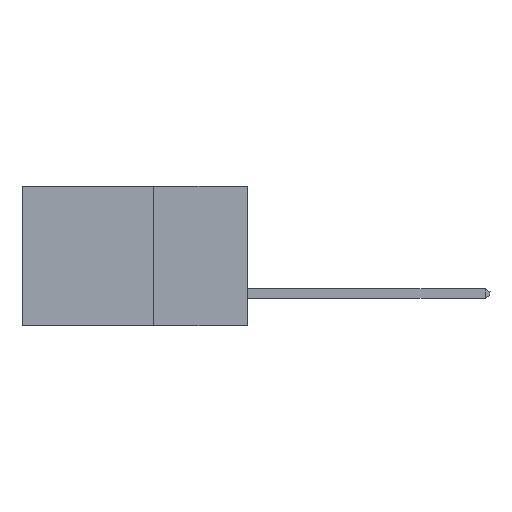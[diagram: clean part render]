
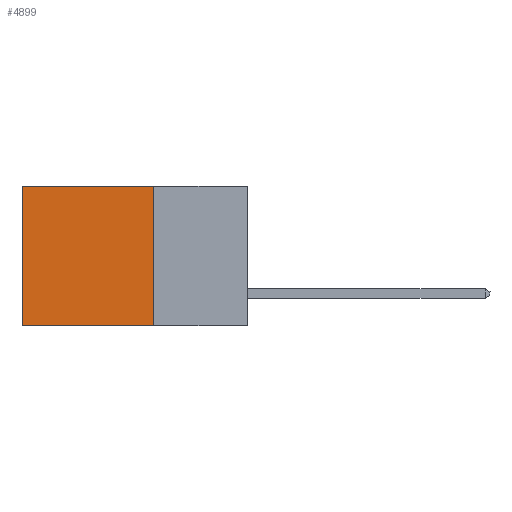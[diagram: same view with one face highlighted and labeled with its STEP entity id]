
A CAD part, left-side view. The second image highlights one B-rep face of the part: STEP entity #4899.
In plain terms, the highlighted planar face has unit normal (-1, 0, 0).
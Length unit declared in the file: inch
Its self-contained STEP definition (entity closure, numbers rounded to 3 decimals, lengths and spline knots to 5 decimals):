
#404 = AXIS2_PLACEMENT_3D ( 'NONE', #7293, #8914, #833 ) ;
#833 = DIRECTION ( 'NONE',  ( 0., 0., -1. ) ) ;
#1270 = CARTESIAN_POINT ( 'NONE',  ( 0.2615, 0.25, 0. ) ) ;
#1564 = FACE_OUTER_BOUND ( 'NONE', #5843, .T. ) ;
#1759 = ORIENTED_EDGE ( 'NONE', *, *, #8696, .T. ) ;
#1832 = VECTOR ( 'NONE', #6645, 39.37008 ) ;
#1913 = ORIENTED_EDGE ( 'NONE', *, *, #4506, .F. ) ;
#1999 = CARTESIAN_POINT ( 'NONE',  ( 0.2615, 0.25, -0.37 ) ) ;
#2515 = EDGE_CURVE ( 'NONE', #5753, #7644, #4645, .T. ) ;
#3374 = EDGE_CURVE ( 'NONE', #5796, #5812, #6791, .T. ) ;
#4292 = VECTOR ( 'NONE', #8492, 39.37008 ) ;
#4506 = EDGE_CURVE ( 'NONE', #5796, #5753, #8198, .T. ) ;
#4645 = LINE ( 'NONE', #7839, #5826 ) ;
#4899 = ADVANCED_FACE ( 'NONE', ( #1564 ), #6525, .F. ) ;
#5390 = DIRECTION ( 'NONE',  ( 0., 0., -1. ) ) ;
#5727 = VECTOR ( 'NONE', #5390, 39.37008 ) ;
#5753 = VERTEX_POINT ( 'NONE', #7578 ) ;
#5796 = VERTEX_POINT ( 'NONE', #1270 ) ;
#5812 = VERTEX_POINT ( 'NONE', #8200 ) ;
#5826 = VECTOR ( 'NONE', #7057, 39.37008 ) ;
#5843 = EDGE_LOOP ( 'NONE', ( #1759, #5981, #1913, #7582 ) ) ;
#5981 = ORIENTED_EDGE ( 'NONE', *, *, #2515, .F. ) ;
#6525 = PLANE ( 'NONE',  #404 ) ;
#6645 = DIRECTION ( 'NONE',  ( 0., 0., -1. ) ) ;
#6746 = CARTESIAN_POINT ( 'NONE',  ( 0.2615, 0.6, -0.37 ) ) ;
#6791 = LINE ( 'NONE', #9162, #4292 ) ;
#6966 = LINE ( 'NONE', #10131, #5727 ) ;
#7057 = DIRECTION ( 'NONE',  ( 0., 1., 0. ) ) ;
#7293 = CARTESIAN_POINT ( 'NONE',  ( 0.2615, 0.25, -0.37 ) ) ;
#7578 = CARTESIAN_POINT ( 'NONE',  ( 0.2615, 0.25, -0.37 ) ) ;
#7582 = ORIENTED_EDGE ( 'NONE', *, *, #3374, .T. ) ;
#7644 = VERTEX_POINT ( 'NONE', #6746 ) ;
#7839 = CARTESIAN_POINT ( 'NONE',  ( 0.2615, 0.25, -0.37 ) ) ;
#8198 = LINE ( 'NONE', #1999, #1832 ) ;
#8200 = CARTESIAN_POINT ( 'NONE',  ( 0.2615, 0.6, 0. ) ) ;
#8492 = DIRECTION ( 'NONE',  ( 0., 1., 0. ) ) ;
#8696 = EDGE_CURVE ( 'NONE', #5812, #7644, #6966, .T. ) ;
#8914 = DIRECTION ( 'NONE',  ( 1., 0., 0. ) ) ;
#9162 = CARTESIAN_POINT ( 'NONE',  ( 0.2615, 0.25, 0. ) ) ;
#10131 = CARTESIAN_POINT ( 'NONE',  ( 0.2615, 0.6, -0.37 ) ) ;
